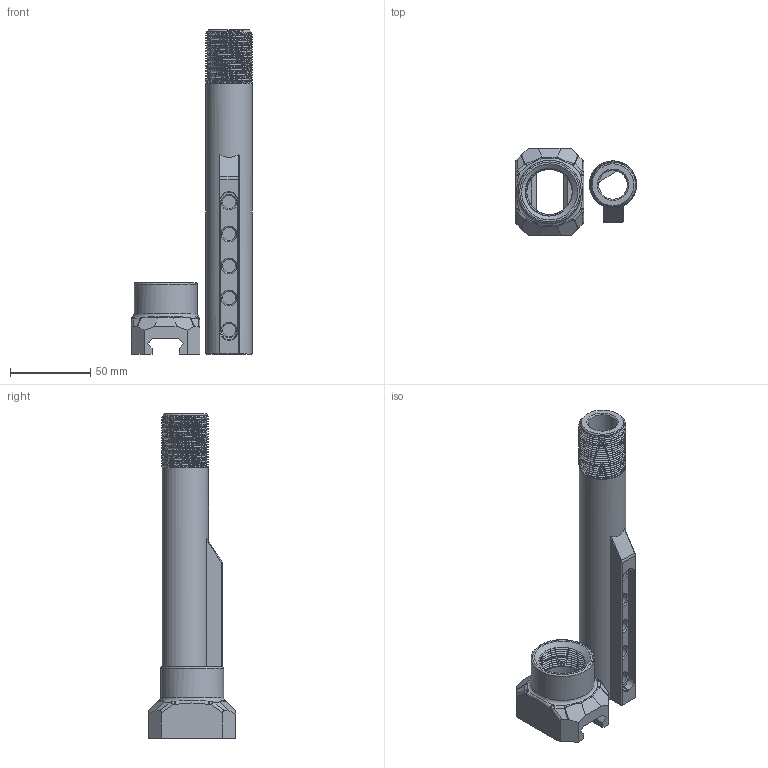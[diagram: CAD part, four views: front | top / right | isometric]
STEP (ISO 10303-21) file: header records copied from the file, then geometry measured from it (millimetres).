
FILE_DESCRIPTION(/* description */ (''),/* implementation_level */ '2;1');
FILE_NAME(/* author */ (''),/* organization */ (''),/* preprocessor_version */ 'ST-DEVELOPER v15.2',/* originating_system */ 'Autodesk Translator Framework v2.0.0.5431',/* authorisation */ '');
FILE_SCHEMA (('AUTOMOTIVE_DESIGN { 1 0 10303 214 3 1 1 }'));
Length unit declared in the file: centimetre
Products named in the file (1): unpublished stocks
Bounding box: 75.64 x 54.44 x 202.53 mm (x, y, z)
Volume: 129406.1 mm3; surface area: 50624.7 mm2
Topology: 2 solids, 2 shells, 190 faces, 587 edges, 407 vertices
Faces by surface type: plane 72, bspline 49, cylinder 47, cone 14, torus 8
Full cylindrical faces by diameter (mm): 8.2 x5, 18 x1, 29 x1, 29.4 x1, 39.4 x1
Entity records: 24872 total; most frequent: CARTESIAN_POINT 20229, ORIENTED_EDGE 1110, DIRECTION 770, EDGE_CURVE 555, VERTEX_POINT 396, AXIS2_PLACEMENT_3D 304, EDGE_LOOP 219, B_SPLINE_CURVE_WITH_KNOTS 208
